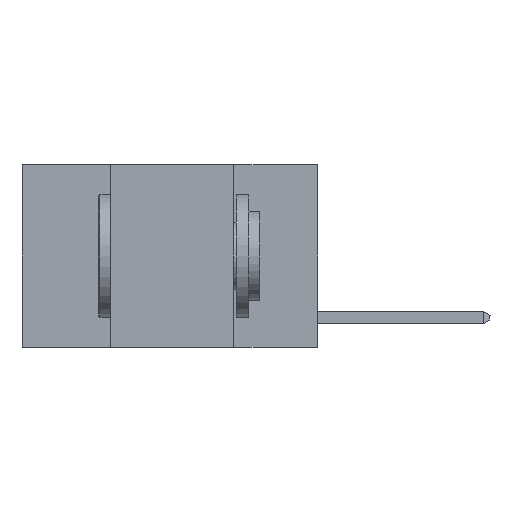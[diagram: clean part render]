
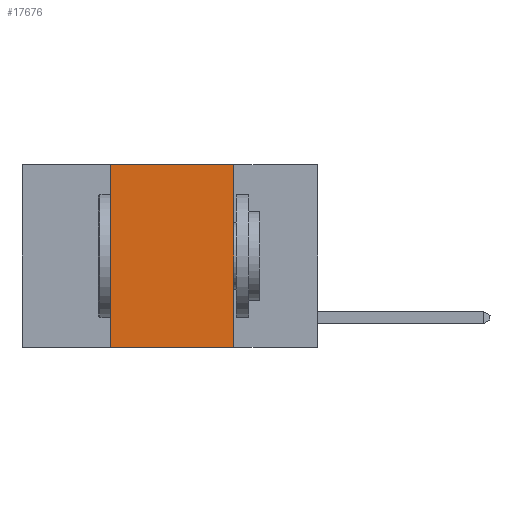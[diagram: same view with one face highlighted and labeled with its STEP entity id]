
A CAD part, left-side view. The second image highlights one B-rep face of the part: STEP entity #17676.
In plain terms, the highlighted planar face has unit normal (-1, 0, 0).
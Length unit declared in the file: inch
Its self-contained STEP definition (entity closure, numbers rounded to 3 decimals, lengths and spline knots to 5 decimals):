
#298 = CARTESIAN_POINT ( 'NONE',  ( 0., 0.42, 0. ) ) ;
#1426 = CARTESIAN_POINT ( 'NONE',  ( 0., 0.6, 0. ) ) ;
#2573 = VECTOR ( 'NONE', #3899, 39.37008 ) ;
#2817 = PLANE ( 'NONE',  #6823 ) ;
#3144 = VECTOR ( 'NONE', #12590, 39.37008 ) ;
#3471 = CARTESIAN_POINT ( 'NONE',  ( 0., 0.42, 0. ) ) ;
#3899 = DIRECTION ( 'NONE',  ( 0., 0., 1. ) ) ;
#3926 = LINE ( 'NONE', #4528, #3144 ) ;
#4070 = VERTEX_POINT ( 'NONE', #8316 ) ;
#4528 = CARTESIAN_POINT ( 'NONE',  ( 0., 0.6, 0. ) ) ;
#4655 = DIRECTION ( 'NONE',  ( 0., 0., -1. ) ) ;
#5444 = VERTEX_POINT ( 'NONE', #18021 ) ;
#6339 = VERTEX_POINT ( 'NONE', #19988 ) ;
#6823 = AXIS2_PLACEMENT_3D ( 'NONE', #1426, #14228, #11305 ) ;
#6970 = FACE_OUTER_BOUND ( 'NONE', #13699, .T. ) ;
#7131 = LINE ( 'NONE', #10915, #18046 ) ;
#7831 = VECTOR ( 'NONE', #4655, 39.37008 ) ;
#8316 = CARTESIAN_POINT ( 'NONE',  ( 0., 0.42, -0.37 ) ) ;
#8521 = ORIENTED_EDGE ( 'NONE', *, *, #18018, .F. ) ;
#9654 = LINE ( 'NONE', #20826, #7831 ) ;
#10082 = EDGE_CURVE ( 'NONE', #4070, #6339, #7131, .T. ) ;
#10915 = CARTESIAN_POINT ( 'NONE',  ( 0., 0.6, -0.37 ) ) ;
#11261 = LINE ( 'NONE', #298, #2573 ) ;
#11305 = DIRECTION ( 'NONE',  ( 0., 0., -1. ) ) ;
#12158 = VERTEX_POINT ( 'NONE', #3471 ) ;
#12377 = EDGE_CURVE ( 'NONE', #12158, #5444, #3926, .T. ) ;
#12590 = DIRECTION ( 'NONE',  ( 0., -1., 0. ) ) ;
#13163 = ORIENTED_EDGE ( 'NONE', *, *, #15134, .F. ) ;
#13699 = EDGE_LOOP ( 'NONE', ( #13163, #14765, #8521, #15001 ) ) ;
#14228 = DIRECTION ( 'NONE',  ( 1., 0., 0. ) ) ;
#14765 = ORIENTED_EDGE ( 'NONE', *, *, #12377, .F. ) ;
#15001 = ORIENTED_EDGE ( 'NONE', *, *, #10082, .T. ) ;
#15134 = EDGE_CURVE ( 'NONE', #5444, #6339, #9654, .T. ) ;
#15828 = DIRECTION ( 'NONE',  ( 0., -1., 0. ) ) ;
#17676 = ADVANCED_FACE ( 'NONE', ( #6970 ), #2817, .F. ) ;
#18018 = EDGE_CURVE ( 'NONE', #4070, #12158, #11261, .T. ) ;
#18021 = CARTESIAN_POINT ( 'NONE',  ( 0., 0.17, 0. ) ) ;
#18046 = VECTOR ( 'NONE', #15828, 39.37008 ) ;
#19988 = CARTESIAN_POINT ( 'NONE',  ( 0., 0.17, -0.37 ) ) ;
#20826 = CARTESIAN_POINT ( 'NONE',  ( 0., 0.17, 0. ) ) ;
